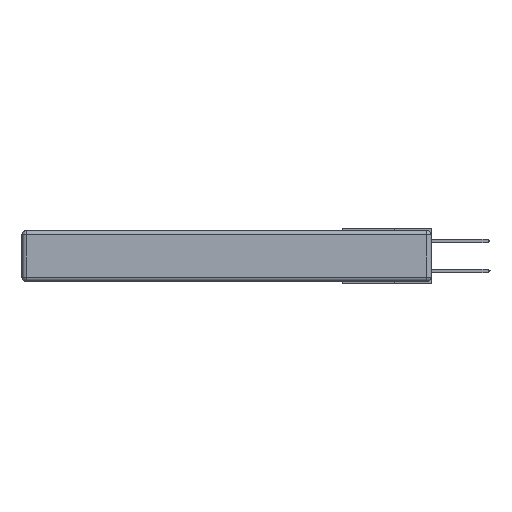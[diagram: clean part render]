
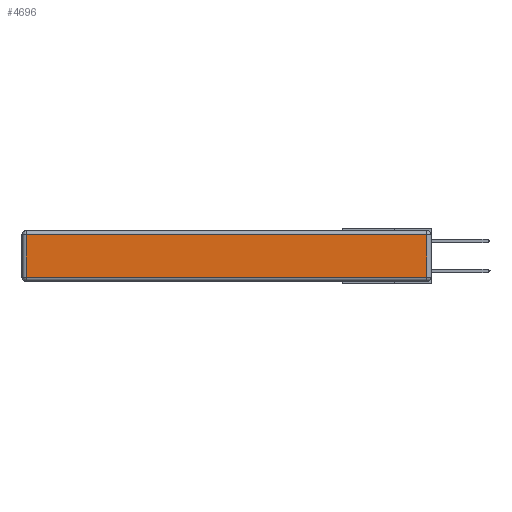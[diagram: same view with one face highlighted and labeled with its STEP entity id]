
A CAD part, left-side view. The second image highlights one B-rep face of the part: STEP entity #4696.
In plain terms, the highlighted planar face has unit normal (-1, 0, 0).
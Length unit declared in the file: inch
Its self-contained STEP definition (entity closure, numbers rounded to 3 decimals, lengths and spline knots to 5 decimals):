
#1431 = VERTEX_POINT ( 'NONE', #3751 ) ;
#2687 = PLANE ( 'NONE',  #6866 ) ;
#2910 = VECTOR ( 'NONE', #8273, 39.37008 ) ;
#3199 = VERTEX_POINT ( 'NONE', #5231 ) ;
#3407 = DIRECTION ( 'NONE',  ( 0., 0., -1. ) ) ;
#3549 = LINE ( 'NONE', #13415, #9826 ) ;
#3751 = CARTESIAN_POINT ( 'NONE',  ( 0., 2.72, -0.03 ) ) ;
#4696 = ADVANCED_FACE ( 'NONE', ( #13246 ), #2687, .T. ) ;
#4910 = CARTESIAN_POINT ( 'NONE',  ( 0., 2.72, -0.343 ) ) ;
#4934 = DIRECTION ( 'NONE',  ( 0., 0., 1. ) ) ;
#5231 = CARTESIAN_POINT ( 'NONE',  ( 0., 0.03, -0.313 ) ) ;
#6312 = VERTEX_POINT ( 'NONE', #8136 ) ;
#6866 = AXIS2_PLACEMENT_3D ( 'NONE', #12654, #13781, #4934 ) ;
#7052 = LINE ( 'NONE', #4910, #10405 ) ;
#7231 = CARTESIAN_POINT ( 'NONE',  ( 0., 0.03, -0.343 ) ) ;
#7332 = EDGE_CURVE ( 'NONE', #3199, #6312, #15877, .T. ) ;
#8136 = CARTESIAN_POINT ( 'NONE',  ( 0., 0.03, -0.03 ) ) ;
#8273 = DIRECTION ( 'NONE',  ( 0., -1., 0. ) ) ;
#8363 = VERTEX_POINT ( 'NONE', #14232 ) ;
#9349 = VECTOR ( 'NONE', #17348, 39.37008 ) ;
#9826 = VECTOR ( 'NONE', #17862, 39.37008 ) ;
#10335 = EDGE_CURVE ( 'NONE', #8363, #3199, #13606, .T. ) ;
#10405 = VECTOR ( 'NONE', #3407, 39.37008 ) ;
#11085 = EDGE_CURVE ( 'NONE', #6312, #1431, #3549, .T. ) ;
#11444 = ORIENTED_EDGE ( 'NONE', *, *, #11085, .T. ) ;
#12654 = CARTESIAN_POINT ( 'NONE',  ( 0., 0., -0.343 ) ) ;
#12804 = ORIENTED_EDGE ( 'NONE', *, *, #7332, .T. ) ;
#13246 = FACE_OUTER_BOUND ( 'NONE', #15594, .T. ) ;
#13415 = CARTESIAN_POINT ( 'NONE',  ( 0., 2.75, -0.03 ) ) ;
#13496 = EDGE_CURVE ( 'NONE', #1431, #8363, #7052, .T. ) ;
#13603 = ORIENTED_EDGE ( 'NONE', *, *, #13496, .T. ) ;
#13606 = LINE ( 'NONE', #13932, #2910 ) ;
#13781 = DIRECTION ( 'NONE',  ( -1., 0., 0. ) ) ;
#13932 = CARTESIAN_POINT ( 'NONE',  ( 0., 0., -0.313 ) ) ;
#14232 = CARTESIAN_POINT ( 'NONE',  ( 0., 2.72, -0.313 ) ) ;
#15594 = EDGE_LOOP ( 'NONE', ( #18439, #12804, #11444, #13603 ) ) ;
#15877 = LINE ( 'NONE', #7231, #9349 ) ;
#17348 = DIRECTION ( 'NONE',  ( 0., 0., 1. ) ) ;
#17862 = DIRECTION ( 'NONE',  ( 0., 1., 0. ) ) ;
#18439 = ORIENTED_EDGE ( 'NONE', *, *, #10335, .T. ) ;
